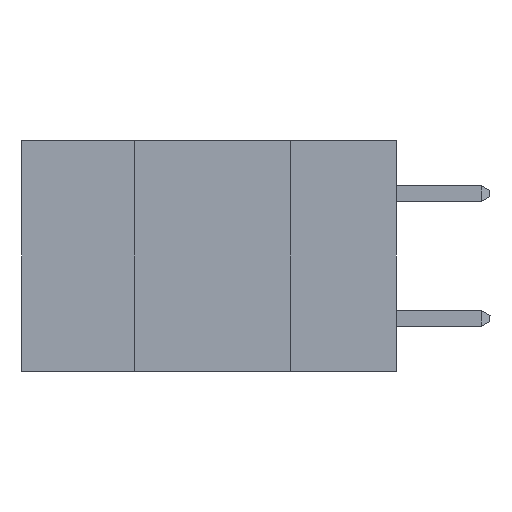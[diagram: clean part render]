
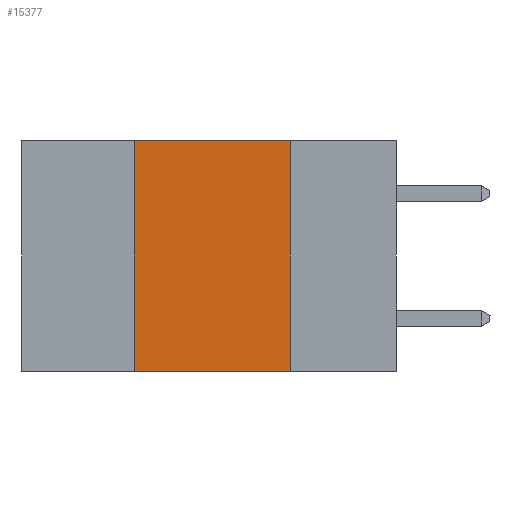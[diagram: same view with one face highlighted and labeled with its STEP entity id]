
A CAD part, left-side view. The second image highlights one B-rep face of the part: STEP entity #15377.
In plain terms, the highlighted planar face has unit normal (-1, 0, 0).
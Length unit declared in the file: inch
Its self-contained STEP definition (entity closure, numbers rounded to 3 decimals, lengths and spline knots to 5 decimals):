
#105 = VECTOR ( 'NONE', #3327, 39.37008 ) ;
#1674 = VECTOR ( 'NONE', #4741, 39.37008 ) ;
#2048 = VECTOR ( 'NONE', #14130, 39.37008 ) ;
#2056 = CARTESIAN_POINT ( 'NONE',  ( 0., 0.17, 0. ) ) ;
#2307 = PLANE ( 'NONE',  #11554 ) ;
#2877 = EDGE_CURVE ( 'NONE', #3263, #4422, #13160, .T. ) ;
#3239 = VERTEX_POINT ( 'NONE', #14403 ) ;
#3247 = LINE ( 'NONE', #7760, #2048 ) ;
#3263 = VERTEX_POINT ( 'NONE', #9444 ) ;
#3327 = DIRECTION ( 'NONE',  ( 0., 0., -1. ) ) ;
#4422 = VERTEX_POINT ( 'NONE', #13246 ) ;
#4596 = CARTESIAN_POINT ( 'NONE',  ( 0., 0.17, 0. ) ) ;
#4741 = DIRECTION ( 'NONE',  ( 0., 0., 1. ) ) ;
#5252 = VERTEX_POINT ( 'NONE', #4596 ) ;
#6648 = ORIENTED_EDGE ( 'NONE', *, *, #10113, .F. ) ;
#6798 = ORIENTED_EDGE ( 'NONE', *, *, #11080, .T. ) ;
#6980 = FACE_OUTER_BOUND ( 'NONE', #9334, .T. ) ;
#7760 = CARTESIAN_POINT ( 'NONE',  ( 0., 0.6, -0.37 ) ) ;
#7898 = ORIENTED_EDGE ( 'NONE', *, *, #2877, .F. ) ;
#9334 = EDGE_LOOP ( 'NONE', ( #6648, #15039, #7898, #6798 ) ) ;
#9444 = CARTESIAN_POINT ( 'NONE',  ( 0., 0.42, -0.37 ) ) ;
#9883 = VECTOR ( 'NONE', #13280, 39.37008 ) ;
#10013 = CARTESIAN_POINT ( 'NONE',  ( 0., 0.6, 0. ) ) ;
#10113 = EDGE_CURVE ( 'NONE', #5252, #3239, #15144, .T. ) ;
#10474 = LINE ( 'NONE', #15745, #9883 ) ;
#11080 = EDGE_CURVE ( 'NONE', #3263, #3239, #3247, .T. ) ;
#11291 = CARTESIAN_POINT ( 'NONE',  ( 0., 0.42, 0. ) ) ;
#11554 = AXIS2_PLACEMENT_3D ( 'NONE', #10013, #13862, #12158 ) ;
#12084 = EDGE_CURVE ( 'NONE', #4422, #5252, #10474, .T. ) ;
#12158 = DIRECTION ( 'NONE',  ( 0., 0., -1. ) ) ;
#13160 = LINE ( 'NONE', #11291, #1674 ) ;
#13246 = CARTESIAN_POINT ( 'NONE',  ( 0., 0.42, 0. ) ) ;
#13280 = DIRECTION ( 'NONE',  ( 0., -1., 0. ) ) ;
#13862 = DIRECTION ( 'NONE',  ( 1., 0., 0. ) ) ;
#14130 = DIRECTION ( 'NONE',  ( 0., -1., 0. ) ) ;
#14403 = CARTESIAN_POINT ( 'NONE',  ( 0., 0.17, -0.37 ) ) ;
#15039 = ORIENTED_EDGE ( 'NONE', *, *, #12084, .F. ) ;
#15144 = LINE ( 'NONE', #2056, #105 ) ;
#15377 = ADVANCED_FACE ( 'NONE', ( #6980 ), #2307, .F. ) ;
#15745 = CARTESIAN_POINT ( 'NONE',  ( 0., 0.6, 0. ) ) ;
